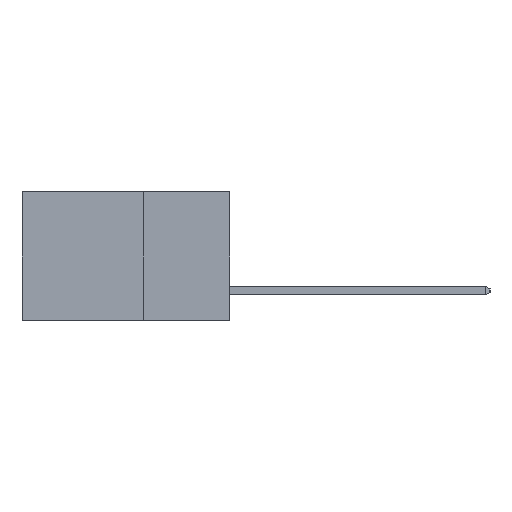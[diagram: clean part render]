
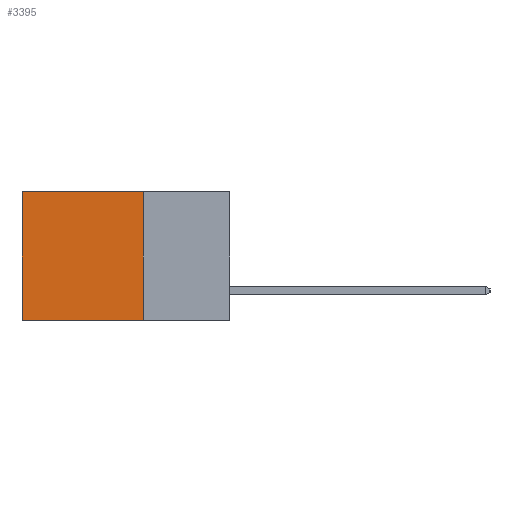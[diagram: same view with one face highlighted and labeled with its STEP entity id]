
A CAD part, left-side view. The second image highlights one B-rep face of the part: STEP entity #3395.
In plain terms, the highlighted planar face has unit normal (-1, 0, 0).
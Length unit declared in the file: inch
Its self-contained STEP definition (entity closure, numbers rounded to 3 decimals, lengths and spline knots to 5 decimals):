
#748 = ORIENTED_EDGE ( 'NONE', *, *, #11885, .F. ) ;
#978 = VECTOR ( 'NONE', #3691, 39.37008 ) ;
#3342 = CARTESIAN_POINT ( 'NONE',  ( 0.2615, 0.25, -0.37 ) ) ;
#3395 = ADVANCED_FACE ( 'NONE', ( #18333 ), #11551, .F. ) ;
#3691 = DIRECTION ( 'NONE',  ( 0., 0., -1. ) ) ;
#3945 = VECTOR ( 'NONE', #6472, 39.37008 ) ;
#4774 = VERTEX_POINT ( 'NONE', #8381 ) ;
#4960 = CARTESIAN_POINT ( 'NONE',  ( 0.2615, 0.25, 0. ) ) ;
#5241 = LINE ( 'NONE', #14679, #978 ) ;
#6472 = DIRECTION ( 'NONE',  ( 0., 1., 0. ) ) ;
#7545 = VECTOR ( 'NONE', #20006, 39.37008 ) ;
#7603 = CARTESIAN_POINT ( 'NONE',  ( 0.2615, 0.25, -0.37 ) ) ;
#7667 = VECTOR ( 'NONE', #7997, 39.37008 ) ;
#7997 = DIRECTION ( 'NONE',  ( 0., 1., 0. ) ) ;
#8102 = LINE ( 'NONE', #3342, #3945 ) ;
#8182 = LINE ( 'NONE', #8989, #7667 ) ;
#8219 = AXIS2_PLACEMENT_3D ( 'NONE', #11524, #11932, #11410 ) ;
#8381 = CARTESIAN_POINT ( 'NONE',  ( 0.2615, 0.6, 0. ) ) ;
#8502 = ORIENTED_EDGE ( 'NONE', *, *, #8833, .T. ) ;
#8780 = ORIENTED_EDGE ( 'NONE', *, *, #20127, .F. ) ;
#8833 = EDGE_CURVE ( 'NONE', #14483, #4774, #8182, .T. ) ;
#8989 = CARTESIAN_POINT ( 'NONE',  ( 0.2615, 0.25, 0. ) ) ;
#10889 = CARTESIAN_POINT ( 'NONE',  ( 0.2615, 0.25, -0.37 ) ) ;
#11410 = DIRECTION ( 'NONE',  ( 0., 0., -1. ) ) ;
#11524 = CARTESIAN_POINT ( 'NONE',  ( 0.2615, 0.25, -0.37 ) ) ;
#11551 = PLANE ( 'NONE',  #8219 ) ;
#11863 = VERTEX_POINT ( 'NONE', #13979 ) ;
#11885 = EDGE_CURVE ( 'NONE', #14483, #14271, #14451, .T. ) ;
#11932 = DIRECTION ( 'NONE',  ( 1., 0., 0. ) ) ;
#13979 = CARTESIAN_POINT ( 'NONE',  ( 0.2615, 0.6, -0.37 ) ) ;
#14271 = VERTEX_POINT ( 'NONE', #7603 ) ;
#14451 = LINE ( 'NONE', #10889, #7545 ) ;
#14483 = VERTEX_POINT ( 'NONE', #4960 ) ;
#14679 = CARTESIAN_POINT ( 'NONE',  ( 0.2615, 0.6, -0.37 ) ) ;
#15398 = EDGE_LOOP ( 'NONE', ( #16220, #8780, #748, #8502 ) ) ;
#16220 = ORIENTED_EDGE ( 'NONE', *, *, #17036, .T. ) ;
#17036 = EDGE_CURVE ( 'NONE', #4774, #11863, #5241, .T. ) ;
#18333 = FACE_OUTER_BOUND ( 'NONE', #15398, .T. ) ;
#20006 = DIRECTION ( 'NONE',  ( 0., 0., -1. ) ) ;
#20127 = EDGE_CURVE ( 'NONE', #14271, #11863, #8102, .T. ) ;
